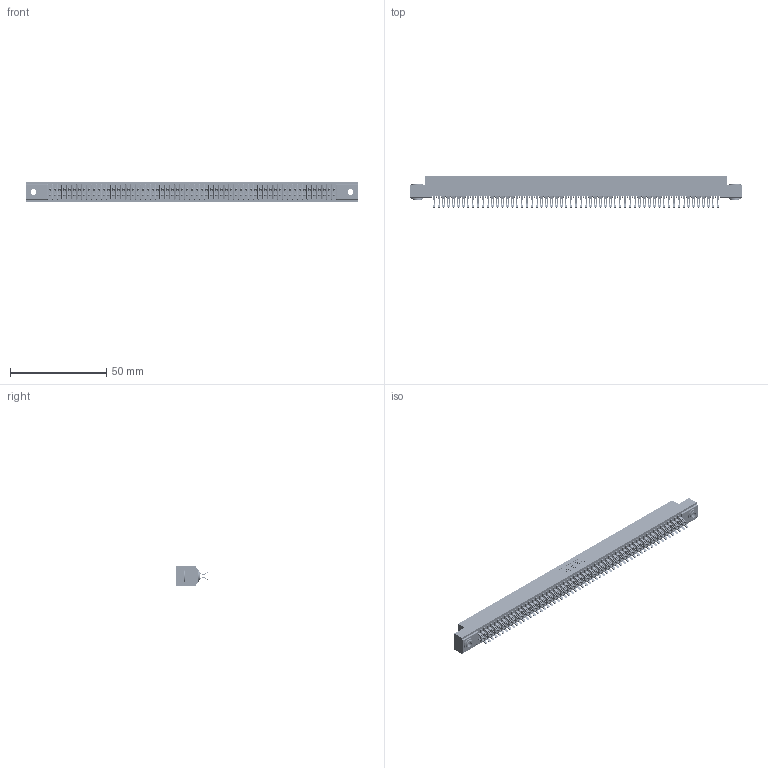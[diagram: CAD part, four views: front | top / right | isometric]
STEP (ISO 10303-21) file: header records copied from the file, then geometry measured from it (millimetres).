
FILE_DESCRIPTION (( 'STEP AP203' ), '1' );
FILE_NAME ('341-118-555-203.STEP', '2018-08-08T14:31:32', ( '' ), ( '' ), 'SwSTEP 2.0', 'SolidWorks 2016', '' );
FILE_SCHEMA (( 'CONFIG_CONTROL_DESIGN' ));
Length unit declared in the file: inch
Products named in the file (4): 341 Part_.156 (3.96) Dia Mounting Holes; 341-292-001_341-292-155; 345-250-002_345-250-002-102; 341-118-555-203
Assembly tree (121 placements, depth 2):
  341-118-555-203
    341 Part_.156 (3.96) Dia Mounting Holes
    341-292-001_341-292-155  x118
    345-250-002_345-250-002-102  x2
Bounding box: 172.09 x 16.31 x 10.16 mm (x, y, z)
Volume: 12873.9 mm3; surface area: 24596.8 mm2
Topology: 121 solids, 121 shells, 9372 faces, 27981 edges, 18214 vertices
Faces by surface type: plane 5048, cylinder 4080, sphere 120, torus 116, cone 8
Entity records: 70673 total; most frequent: CARTESIAN_POINT 11744, ORIENTED_EDGE 11654, DIRECTION 11391, EDGE_CURVE 5827, VECTOR 4701, LINE 4701, VERTEX_POINT 3682, AXIS2_PLACEMENT_3D 3345
